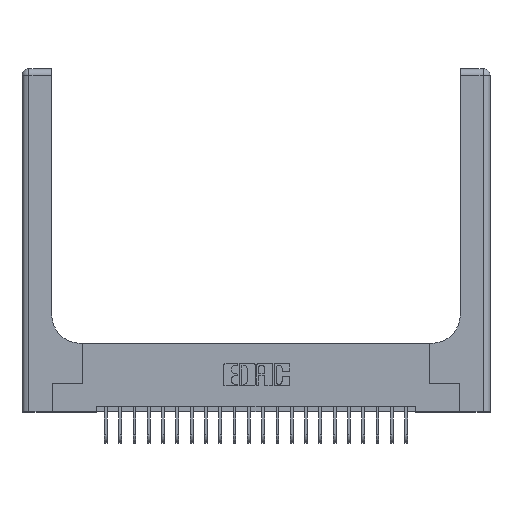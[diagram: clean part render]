
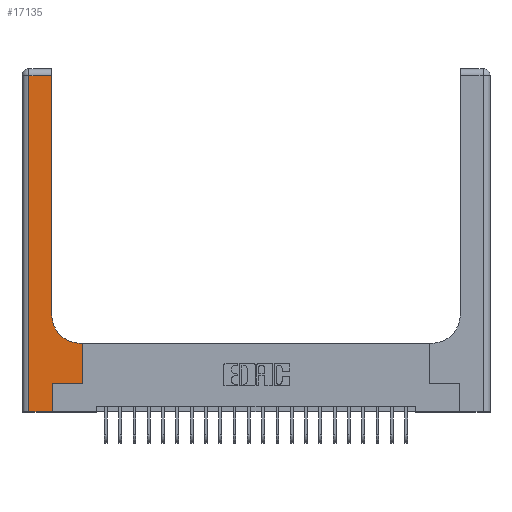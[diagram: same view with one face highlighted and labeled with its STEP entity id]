
A CAD part, top view. The second image highlights one B-rep face of the part: STEP entity #17135.
In plain terms, the highlighted planar face has unit normal (0, 0, 1).
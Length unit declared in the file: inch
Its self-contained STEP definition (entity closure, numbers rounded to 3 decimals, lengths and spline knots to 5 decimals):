
#6 = VECTOR ( 'NONE', #8477, 39.37008 ) ;
#532 = EDGE_CURVE ( 'NONE', #13771, #3347, #13953, .T. ) ;
#562 = EDGE_LOOP ( 'NONE', ( #10877, #12453, #6973, #19424, #19926, #17129, #18858, #12434, #2469 ) ) ;
#718 = VERTEX_POINT ( 'NONE', #3413 ) ;
#900 = DIRECTION ( 'NONE',  ( -1., 0., 0. ) ) ;
#1697 = CARTESIAN_POINT ( 'NONE',  ( 0., 3., 0.37 ) ) ;
#2469 = ORIENTED_EDGE ( 'NONE', *, *, #21264, .T. ) ;
#3189 = VERTEX_POINT ( 'NONE', #15975 ) ;
#3347 = VERTEX_POINT ( 'NONE', #13251 ) ;
#3413 = CARTESIAN_POINT ( 'NONE',  ( 0.06, 2.94, 0.37 ) ) ;
#3805 = VERTEX_POINT ( 'NONE', #7160 ) ;
#4075 = DIRECTION ( 'NONE',  ( 0., 0., -1. ) ) ;
#4267 = CARTESIAN_POINT ( 'NONE',  ( 0.265, 0., 0.37 ) ) ;
#4369 = CARTESIAN_POINT ( 'NONE',  ( 0.528, 0.6, 0.37 ) ) ;
#6279 = LINE ( 'NONE', #19630, #10699 ) ;
#6393 = EDGE_CURVE ( 'NONE', #718, #16243, #7264, .T. ) ;
#6578 = AXIS2_PLACEMENT_3D ( 'NONE', #1697, #18450, #8541 ) ;
#6722 = DIRECTION ( 'NONE',  ( 0., -1., 0. ) ) ;
#6736 = EDGE_CURVE ( 'NONE', #16243, #3189, #18151, .T. ) ;
#6842 = PLANE ( 'NONE',  #6578 ) ;
#6900 = VECTOR ( 'NONE', #20062, 39.37008 ) ;
#6973 = ORIENTED_EDGE ( 'NONE', *, *, #6393, .T. ) ;
#6994 = CARTESIAN_POINT ( 'NONE',  ( 0.51, 0.6, 0.37 ) ) ;
#7160 = CARTESIAN_POINT ( 'NONE',  ( 0.26, 2.94, 0.37 ) ) ;
#7264 = LINE ( 'NONE', #21550, #11145 ) ;
#7559 = VECTOR ( 'NONE', #900, 39.37008 ) ;
#7677 = CARTESIAN_POINT ( 'NONE',  ( 0., 0., 0.37 ) ) ;
#8074 = DIRECTION ( 'NONE',  ( -1., 0., 0. ) ) ;
#8127 = EDGE_CURVE ( 'NONE', #8151, #3805, #20114, .T. ) ;
#8151 = VERTEX_POINT ( 'NONE', #20586 ) ;
#8477 = DIRECTION ( 'NONE',  ( 1., 0., 0. ) ) ;
#8540 = EDGE_CURVE ( 'NONE', #3347, #16787, #15721, .T. ) ;
#8541 = DIRECTION ( 'NONE',  ( -1., 0., 0. ) ) ;
#8546 = CARTESIAN_POINT ( 'NONE',  ( 0.265, 0.25, 0.37 ) ) ;
#9329 = CARTESIAN_POINT ( 'NONE',  ( 0.26, 0.6, 0.37 ) ) ;
#9811 = LINE ( 'NONE', #4267, #15240 ) ;
#9848 = VECTOR ( 'NONE', #19266, 39.37008 ) ;
#10118 = FACE_OUTER_BOUND ( 'NONE', #562, .T. ) ;
#10699 = VECTOR ( 'NONE', #8074, 39.37008 ) ;
#10877 = ORIENTED_EDGE ( 'NONE', *, *, #8127, .T. ) ;
#11145 = VECTOR ( 'NONE', #6722, 39.37008 ) ;
#11161 = CARTESIAN_POINT ( 'NONE',  ( 0.06, 0., 0.37 ) ) ;
#11425 = EDGE_CURVE ( 'NONE', #3805, #718, #6279, .T. ) ;
#11935 = AXIS2_PLACEMENT_3D ( 'NONE', #14070, #4075, #15710 ) ;
#12300 = DIRECTION ( 'NONE',  ( 0., 1., 0. ) ) ;
#12434 = ORIENTED_EDGE ( 'NONE', *, *, #17477, .T. ) ;
#12453 = ORIENTED_EDGE ( 'NONE', *, *, #11425, .T. ) ;
#12488 = LINE ( 'NONE', #9329, #7559 ) ;
#13251 = CARTESIAN_POINT ( 'NONE',  ( 0.528, 0.25, 0.37 ) ) ;
#13373 = CARTESIAN_POINT ( 'NONE',  ( 0.265, 0.25, 0.37 ) ) ;
#13444 = CARTESIAN_POINT ( 'NONE',  ( 0.528, 0.25, 0.37 ) ) ;
#13771 = VERTEX_POINT ( 'NONE', #13373 ) ;
#13953 = LINE ( 'NONE', #8546, #6 ) ;
#14070 = CARTESIAN_POINT ( 'NONE',  ( 0.51, 0.85, 0.37 ) ) ;
#14072 = EDGE_CURVE ( 'NONE', #3189, #13771, #9811, .T. ) ;
#14882 = CIRCLE ( 'NONE', #11935, 0.25 ) ;
#15009 = VERTEX_POINT ( 'NONE', #6994 ) ;
#15240 = VECTOR ( 'NONE', #20784, 39.37008 ) ;
#15553 = CARTESIAN_POINT ( 'NONE',  ( 0.26, 3., 0.37 ) ) ;
#15710 = DIRECTION ( 'NONE',  ( 1., 0., 0. ) ) ;
#15721 = LINE ( 'NONE', #13444, #6900 ) ;
#15975 = CARTESIAN_POINT ( 'NONE',  ( 0.265, 0., 0.37 ) ) ;
#16243 = VERTEX_POINT ( 'NONE', #11161 ) ;
#16787 = VERTEX_POINT ( 'NONE', #4369 ) ;
#17129 = ORIENTED_EDGE ( 'NONE', *, *, #532, .T. ) ;
#17135 = ADVANCED_FACE ( 'NONE', ( #10118 ), #6842, .F. ) ;
#17477 = EDGE_CURVE ( 'NONE', #16787, #15009, #12488, .T. ) ;
#18151 = LINE ( 'NONE', #7677, #9848 ) ;
#18450 = DIRECTION ( 'NONE',  ( 0., 0., -1. ) ) ;
#18858 = ORIENTED_EDGE ( 'NONE', *, *, #8540, .T. ) ;
#19127 = VECTOR ( 'NONE', #12300, 39.37008 ) ;
#19266 = DIRECTION ( 'NONE',  ( 1., 0., 0. ) ) ;
#19424 = ORIENTED_EDGE ( 'NONE', *, *, #6736, .T. ) ;
#19630 = CARTESIAN_POINT ( 'NONE',  ( 0., 2.94, 0.37 ) ) ;
#19926 = ORIENTED_EDGE ( 'NONE', *, *, #14072, .T. ) ;
#20062 = DIRECTION ( 'NONE',  ( 0., 1., 0. ) ) ;
#20114 = LINE ( 'NONE', #15553, #19127 ) ;
#20586 = CARTESIAN_POINT ( 'NONE',  ( 0.26, 0.85, 0.37 ) ) ;
#20784 = DIRECTION ( 'NONE',  ( 0., 1., 0. ) ) ;
#21264 = EDGE_CURVE ( 'NONE', #15009, #8151, #14882, .T. ) ;
#21550 = CARTESIAN_POINT ( 'NONE',  ( 0.06, 3., 0.37 ) ) ;
